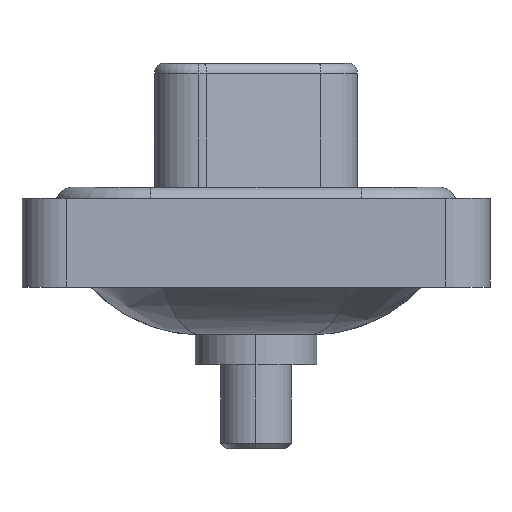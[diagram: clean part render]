
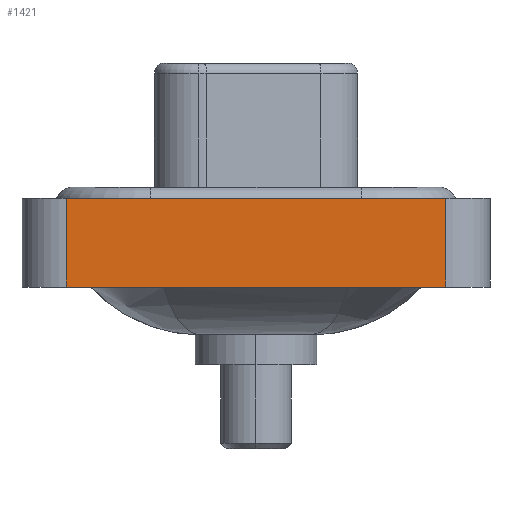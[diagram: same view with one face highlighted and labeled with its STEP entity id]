
A CAD part, left-side view. The second image highlights one B-rep face of the part: STEP entity #1421.
In plain terms, the highlighted planar face has unit normal (-1, 0, 0).
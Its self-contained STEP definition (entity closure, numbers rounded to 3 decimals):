
#1421 = ADVANCED_FACE ( 'NONE', ( #6942 ), #3138, .T. ) ;
#1646 = CARTESIAN_POINT ( 'NONE',  ( -7.3, -8.55, -3.6 ) ) ;
#3138 = PLANE ( 'NONE',  #5863 ) ;
#3394 = DIRECTION ( 'NONE',  ( -1., 0., 0. ) ) ;
#4103 = DIRECTION ( 'NONE',  ( 0., 0., 1. ) ) ;
#4489 = EDGE_CURVE ( 'NONE', #14149, #14043, #5866, .T. ) ;
#5033 = LINE ( 'NONE', #7487, #12702 ) ;
#5373 = CARTESIAN_POINT ( 'NONE',  ( -7.3, 8.55, -3.6 ) ) ;
#5863 = AXIS2_PLACEMENT_3D ( 'NONE', #7188, #3394, #8382 ) ;
#5866 = LINE ( 'NONE', #11002, #14021 ) ;
#6107 = EDGE_CURVE ( 'NONE', #6937, #14149, #13060, .T. ) ;
#6316 = ORIENTED_EDGE ( 'NONE', *, *, #6107, .F. ) ;
#6894 = LINE ( 'NONE', #1646, #16714 ) ;
#6937 = VERTEX_POINT ( 'NONE', #15397 ) ;
#6942 = FACE_OUTER_BOUND ( 'NONE', #13354, .T. ) ;
#7188 = CARTESIAN_POINT ( 'NONE',  ( -7.3, -8.55, -3.6 ) ) ;
#7487 = CARTESIAN_POINT ( 'NONE',  ( -7.3, -8.55, -3.6 ) ) ;
#8054 = CARTESIAN_POINT ( 'NONE',  ( -7.3, 8.55, 0.4 ) ) ;
#8282 = ORIENTED_EDGE ( 'NONE', *, *, #15563, .T. ) ;
#8382 = DIRECTION ( 'NONE',  ( 0., 0., 1. ) ) ;
#8675 = ORIENTED_EDGE ( 'NONE', *, *, #12798, .T. ) ;
#8936 = CARTESIAN_POINT ( 'NONE',  ( -7.3, -8.55, 0.4 ) ) ;
#9326 = ORIENTED_EDGE ( 'NONE', *, *, #4489, .F. ) ;
#9604 = CARTESIAN_POINT ( 'NONE',  ( -7.3, -8.55, -3.6 ) ) ;
#10182 = DIRECTION ( 'NONE',  ( 0., 0., 1. ) ) ;
#11002 = CARTESIAN_POINT ( 'NONE',  ( -7.3, -8.55, 0.4 ) ) ;
#11324 = VECTOR ( 'NONE', #4103, 1000. ) ;
#12702 = VECTOR ( 'NONE', #10182, 1000. ) ;
#12798 = EDGE_CURVE ( 'NONE', #13891, #14043, #5033, .T. ) ;
#13060 = LINE ( 'NONE', #5373, #11324 ) ;
#13354 = EDGE_LOOP ( 'NONE', ( #8675, #9326, #6316, #8282 ) ) ;
#13633 = DIRECTION ( 'NONE',  ( 0., -1., 0. ) ) ;
#13891 = VERTEX_POINT ( 'NONE', #9604 ) ;
#14021 = VECTOR ( 'NONE', #13633, 1000. ) ;
#14043 = VERTEX_POINT ( 'NONE', #8936 ) ;
#14149 = VERTEX_POINT ( 'NONE', #8054 ) ;
#15397 = CARTESIAN_POINT ( 'NONE',  ( -7.3, 8.55, -3.6 ) ) ;
#15563 = EDGE_CURVE ( 'NONE', #6937, #13891, #6894, .T. ) ;
#15669 = DIRECTION ( 'NONE',  ( 0., -1., 0. ) ) ;
#16714 = VECTOR ( 'NONE', #15669, 1000. ) ;
